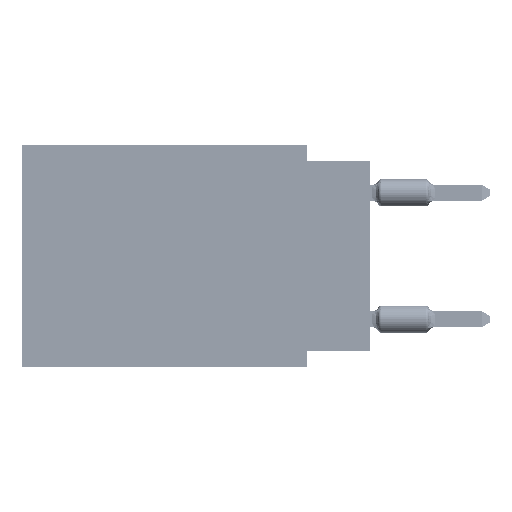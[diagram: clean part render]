
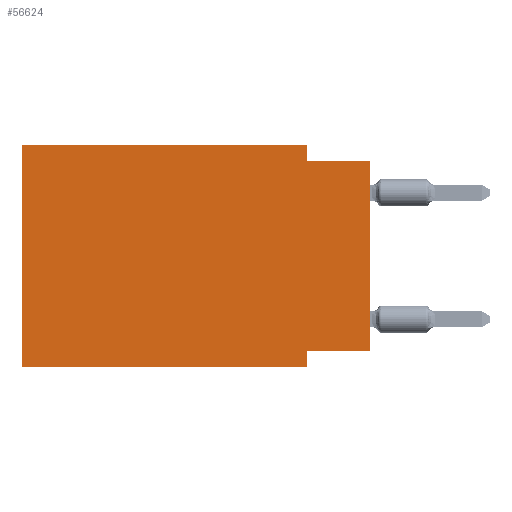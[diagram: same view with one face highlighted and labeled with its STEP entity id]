
A CAD part, left-side view. The second image highlights one B-rep face of the part: STEP entity #56624.
In plain terms, the highlighted planar face has unit normal (-1, 0, 0).
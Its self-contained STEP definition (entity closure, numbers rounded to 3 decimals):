
#422 = AXIS2_PLACEMENT_3D ( 'NONE', #72516, #17198, #51793 ) ;
#2406 = DIRECTION ( 'NONE',  ( 0., -1., 0. ) ) ;
#5966 = CARTESIAN_POINT ( 'NONE',  ( 0., 0., 0. ) ) ;
#7743 = VERTEX_POINT ( 'NONE', #22483 ) ;
#10069 = CARTESIAN_POINT ( 'NONE',  ( 0., 13.97, -8.89 ) ) ;
#11358 = LINE ( 'NONE', #39470, #30317 ) ;
#11905 = ORIENTED_EDGE ( 'NONE', *, *, #15957, .F. ) ;
#13267 = CARTESIAN_POINT ( 'NONE',  ( 0., 2.54, 0. ) ) ;
#15177 = CARTESIAN_POINT ( 'NONE',  ( 0., 13.97, 0. ) ) ;
#15957 = EDGE_CURVE ( 'NONE', #62296, #60408, #47073, .T. ) ;
#17188 = EDGE_LOOP ( 'NONE', ( #18520, #90109, #11905, #41666, #25145, #40018, #84138, #84788 ) ) ;
#17198 = DIRECTION ( 'NONE',  ( 1., 0., 0. ) ) ;
#18520 = ORIENTED_EDGE ( 'NONE', *, *, #68407, .T. ) ;
#18535 = VERTEX_POINT ( 'NONE', #90561 ) ;
#18962 = CARTESIAN_POINT ( 'NONE',  ( 0., 2.54, -8.89 ) ) ;
#22483 = CARTESIAN_POINT ( 'NONE',  ( 0., 2.54, -8.255 ) ) ;
#23667 = FACE_OUTER_BOUND ( 'NONE', #17188, .T. ) ;
#24055 = DIRECTION ( 'NONE',  ( 0., 0., -1. ) ) ;
#24805 = LINE ( 'NONE', #10069, #73059 ) ;
#24985 = EDGE_CURVE ( 'NONE', #60408, #72478, #49474, .T. ) ;
#25145 = ORIENTED_EDGE ( 'NONE', *, *, #52902, .F. ) ;
#26587 = CARTESIAN_POINT ( 'NONE',  ( 0., 13.97, 0. ) ) ;
#28525 = CARTESIAN_POINT ( 'NONE',  ( 0., 13.97, -8.89 ) ) ;
#30317 = VECTOR ( 'NONE', #31611, 1000. ) ;
#31611 = DIRECTION ( 'NONE',  ( 0., 1., 0. ) ) ;
#33249 = VECTOR ( 'NONE', #65378, 1000. ) ;
#36014 = EDGE_CURVE ( 'NONE', #82214, #18535, #24805, .T. ) ;
#39470 = CARTESIAN_POINT ( 'NONE',  ( 0., 0., -8.255 ) ) ;
#40018 = ORIENTED_EDGE ( 'NONE', *, *, #36014, .T. ) ;
#41666 = ORIENTED_EDGE ( 'NONE', *, *, #89726, .F. ) ;
#47073 = LINE ( 'NONE', #53081, #54749 ) ;
#49474 = LINE ( 'NONE', #65543, #54362 ) ;
#51793 = DIRECTION ( 'NONE',  ( 0., 0., -1. ) ) ;
#52218 = PLANE ( 'NONE',  #422 ) ;
#52902 = EDGE_CURVE ( 'NONE', #82214, #57607, #72301, .T. ) ;
#53081 = CARTESIAN_POINT ( 'NONE',  ( 0., 2.54, 0. ) ) ;
#54067 = VECTOR ( 'NONE', #76358, 1000. ) ;
#54362 = VECTOR ( 'NONE', #2406, 1000. ) ;
#54749 = VECTOR ( 'NONE', #24055, 1000. ) ;
#56211 = LINE ( 'NONE', #5966, #87384 ) ;
#56624 = ADVANCED_FACE ( 'NONE', ( #23667 ), #52218, .F. ) ;
#57607 = VERTEX_POINT ( 'NONE', #57682 ) ;
#57682 = CARTESIAN_POINT ( 'NONE',  ( 0., 13.97, 0. ) ) ;
#60408 = VERTEX_POINT ( 'NONE', #69850 ) ;
#61194 = VECTOR ( 'NONE', #61359, 1000. ) ;
#61359 = DIRECTION ( 'NONE',  ( 0., 0., -1. ) ) ;
#62282 = VERTEX_POINT ( 'NONE', #83781 ) ;
#62296 = VERTEX_POINT ( 'NONE', #13267 ) ;
#65378 = DIRECTION ( 'NONE',  ( 0., 0., 1. ) ) ;
#65543 = CARTESIAN_POINT ( 'NONE',  ( 0., 0., -0.635 ) ) ;
#66129 = CARTESIAN_POINT ( 'NONE',  ( 0., 0., -0.635 ) ) ;
#68407 = EDGE_CURVE ( 'NONE', #62282, #72478, #56211, .T. ) ;
#69850 = CARTESIAN_POINT ( 'NONE',  ( 0., 2.54, -0.635 ) ) ;
#70942 = EDGE_CURVE ( 'NONE', #7743, #18535, #75178, .T. ) ;
#72301 = LINE ( 'NONE', #15177, #33249 ) ;
#72478 = VERTEX_POINT ( 'NONE', #66129 ) ;
#72516 = CARTESIAN_POINT ( 'NONE',  ( 0., 13.97, 0. ) ) ;
#73059 = VECTOR ( 'NONE', #79208, 1000. ) ;
#73066 = EDGE_CURVE ( 'NONE', #62282, #7743, #11358, .T. ) ;
#75178 = LINE ( 'NONE', #18962, #61194 ) ;
#75875 = LINE ( 'NONE', #26587, #54067 ) ;
#76358 = DIRECTION ( 'NONE',  ( 0., -1., 0. ) ) ;
#79208 = DIRECTION ( 'NONE',  ( 0., -1., 0. ) ) ;
#82214 = VERTEX_POINT ( 'NONE', #28525 ) ;
#83781 = CARTESIAN_POINT ( 'NONE',  ( 0., 0., -8.255 ) ) ;
#84138 = ORIENTED_EDGE ( 'NONE', *, *, #70942, .F. ) ;
#84788 = ORIENTED_EDGE ( 'NONE', *, *, #73066, .F. ) ;
#87384 = VECTOR ( 'NONE', #89398, 1000. ) ;
#89398 = DIRECTION ( 'NONE',  ( 0., 0., 1. ) ) ;
#89726 = EDGE_CURVE ( 'NONE', #57607, #62296, #75875, .T. ) ;
#90109 = ORIENTED_EDGE ( 'NONE', *, *, #24985, .F. ) ;
#90561 = CARTESIAN_POINT ( 'NONE',  ( 0., 2.54, -8.89 ) ) ;
